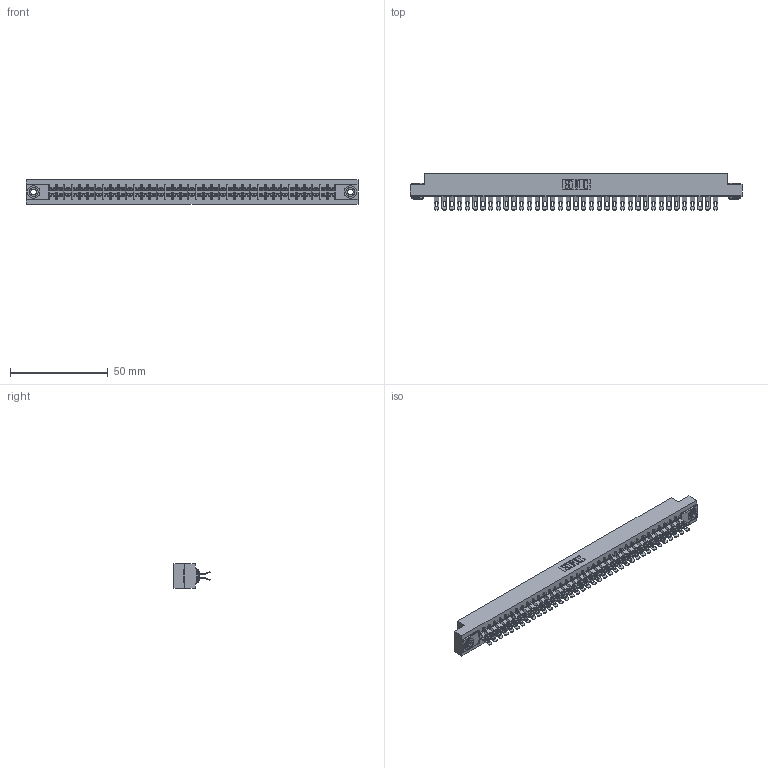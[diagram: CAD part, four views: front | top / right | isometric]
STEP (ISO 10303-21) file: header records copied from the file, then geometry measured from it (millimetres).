
FILE_DESCRIPTION (( 'STEP AP203' ), '1' );
FILE_NAME ('355-074-555-503.STEP', '2019-09-13T12:51:28', ( '' ), ( '' ), 'SwSTEP 2.0', 'SolidWorks 2016', '' );
FILE_SCHEMA (( 'CONFIG_CONTROL_DESIGN' ));
Length unit declared in the file: inch
Products named in the file (4): 305 Part_.156 Dia; 305-290-001_555; 345-250-002_345-250-002-102; 355-074-555-503
Assembly tree (77 placements, depth 2):
  355-074-555-503
    305 Part_.156 Dia
    305-290-001_555  x74
    345-250-002_345-250-002-102  x2
Bounding box: 169.62 x 18.41 x 12.7 mm (x, y, z)
Volume: 17373.7 mm3; surface area: 24452.2 mm2
Topology: 77 solids, 77 shells, 5052 faces, 15043 edges, 9826 vertices
Faces by surface type: plane 2460, cylinder 2436, sphere 148, cone 8
Entity records: 42359 total; most frequent: CARTESIAN_POINT 7008, ORIENTED_EDGE 6938, DIRECTION 6793, EDGE_CURVE 3469, VECTOR 2771, LINE 2771, VERTEX_POINT 2210, AXIS2_PLACEMENT_3D 2011
